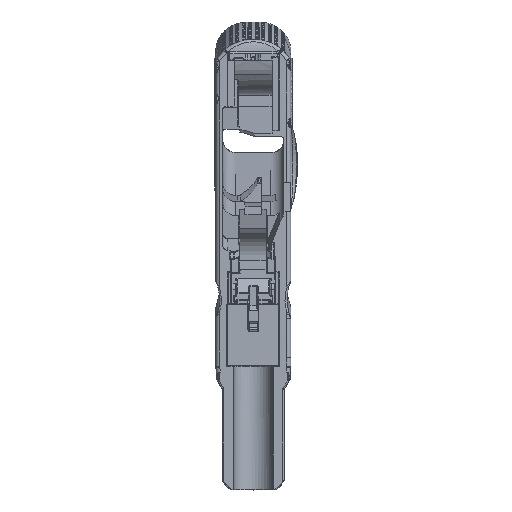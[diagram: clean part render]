
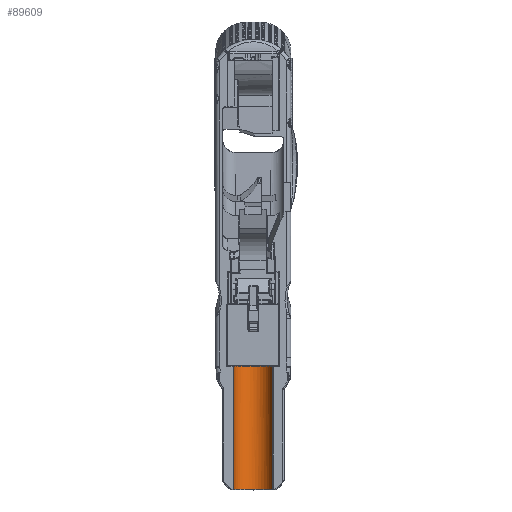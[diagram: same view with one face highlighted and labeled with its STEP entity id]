
A CAD part, top view. The second image highlights one B-rep face of the part: STEP entity #89609.
In plain terms, the highlighted cylindrical face has radius 7.62 mm (diameter 15.24 mm), a partial arc.
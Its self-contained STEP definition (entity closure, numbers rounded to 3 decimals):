
#1249=CYLINDRICAL_SURFACE('',#95398,7.62);
#2247=CIRCLE('',#94868,7.62);
#2250=CIRCLE('',#94872,7.62);
#2254=CIRCLE('',#94876,7.62);
#2475=CIRCLE('',#95399,7.62);
#4872=FACE_OUTER_BOUND('',#10265,.T.);
#10265=EDGE_LOOP('',(#61090,#61091,#61092,#61093,#61094,#61095,#61096,#61097));
#15929=B_SPLINE_CURVE_WITH_KNOTS('',3,(#133860,#133861,#133862,#133863),
 .UNSPECIFIED.,.F.,.F.,(4,4),(0.,0.1),.UNSPECIFIED.);
#15996=B_SPLINE_CURVE_WITH_KNOTS('',3,(#139963,#139964,#139965,#139966),
 .UNSPECIFIED.,.F.,.F.,(4,4),(-0.1,0.),.UNSPECIFIED.);
#18029=LINE('',#138483,#27326);
#18118=LINE('',#139979,#27415);
#27326=VECTOR('',#104218,10.);
#27415=VECTOR('',#104623,10.);
#36746=VERTEX_POINT('',#132628);
#36834=VERTEX_POINT('',#133801);
#36835=VERTEX_POINT('',#133803);
#36836=VERTEX_POINT('',#133808);
#36837=VERTEX_POINT('',#133831);
#37235=VERTEX_POINT('',#138482);
#37351=VERTEX_POINT('',#139960);
#37355=VERTEX_POINT('',#139978);
#45784=EDGE_CURVE('',#36834,#36835,#2247,.T.);
#45787=EDGE_CURVE('',#36835,#36836,#2250,.T.);
#45791=EDGE_CURVE('',#36836,#36837,#2254,.T.);
#45793=EDGE_CURVE('',#36837,#36746,#15929,.T.);
#46393=EDGE_CURVE('',#36746,#37235,#18029,.T.);
#46598=EDGE_CURVE('',#37351,#36834,#15996,.T.);
#46603=EDGE_CURVE('',#37355,#37351,#18118,.T.);
#46604=EDGE_CURVE('',#37235,#37355,#2475,.T.);
#61090=ORIENTED_EDGE('',*,*,#46603,.F.);
#61091=ORIENTED_EDGE('',*,*,#46604,.F.);
#61092=ORIENTED_EDGE('',*,*,#46393,.F.);
#61093=ORIENTED_EDGE('',*,*,#45793,.F.);
#61094=ORIENTED_EDGE('',*,*,#45791,.F.);
#61095=ORIENTED_EDGE('',*,*,#45787,.F.);
#61096=ORIENTED_EDGE('',*,*,#45784,.F.);
#61097=ORIENTED_EDGE('',*,*,#46598,.F.);
#89609=ADVANCED_FACE('',(#4872),#1249,.F.);
#94868=AXIS2_PLACEMENT_3D('',#133804,#103093,#103094);
#94872=AXIS2_PLACEMENT_3D('',#133809,#103101,#103102);
#94876=AXIS2_PLACEMENT_3D('',#133835,#103109,#103110);
#95398=AXIS2_PLACEMENT_3D('',#139977,#104621,#104622);
#95399=AXIS2_PLACEMENT_3D('',#139980,#104624,#104625);
#103093=DIRECTION('center_axis',(0.04,0.999,-0.013));
#103094=DIRECTION('ref_axis',(0.949,-0.042,-0.313));
#103101=DIRECTION('center_axis',(0.,1.,0.));
#103102=DIRECTION('ref_axis',(0.,0.,
-1.));
#103109=DIRECTION('center_axis',(-0.04,0.999,
-0.013));
#103110=DIRECTION('ref_axis',(-0.991,-0.041,-0.127));
#104218=DIRECTION('',(0.,1.,0.));
#104621=DIRECTION('center_axis',(0.,1.,0.));
#104622=DIRECTION('ref_axis',(1.,0.,0.));
#104623=DIRECTION('',(0.,-1.,0.));
#104624=DIRECTION('center_axis',(0.,-1.,0.));
#104625=DIRECTION('ref_axis',(0.,0.,
-1.));
#132628=CARTESIAN_POINT('',(-7.62,-74.215,70.65));
#133801=CARTESIAN_POINT('',(7.558,-74.219,69.684));
#133803=CARTESIAN_POINT('',(7.236,-74.225,68.261));
#133804=CARTESIAN_POINT('Origin',(0.007,-73.908,
70.647));
#133808=CARTESIAN_POINT('',(-7.236,-74.225,68.262));
#133809=CARTESIAN_POINT('Origin',(0.,-74.225,
70.65));
#133831=CARTESIAN_POINT('',(-7.558,-74.219,69.684));
#133835=CARTESIAN_POINT('Origin',(-0.006,-73.908,
70.647));
#133860=CARTESIAN_POINT('Ctrl Pts',(-7.558,-74.219,
69.684));
#133861=CARTESIAN_POINT('Ctrl Pts',(-7.599,-74.217,
70.004));
#133862=CARTESIAN_POINT('Ctrl Pts',(-7.62,-74.215,
70.327));
#133863=CARTESIAN_POINT('Ctrl Pts',(-7.62,-74.215,
70.65));
#138482=CARTESIAN_POINT('',(-7.62,-26.317,70.65));
#138483=CARTESIAN_POINT('',(-7.62,-74.479,70.65));
#139960=CARTESIAN_POINT('',(7.62,-74.215,70.65));
#139963=CARTESIAN_POINT('Ctrl Pts',(7.62,-74.215,70.65));
#139964=CARTESIAN_POINT('Ctrl Pts',(7.62,-74.215,70.327));
#139965=CARTESIAN_POINT('Ctrl Pts',(7.599,-74.217,70.004));
#139966=CARTESIAN_POINT('Ctrl Pts',(7.558,-74.219,69.684));
#139977=CARTESIAN_POINT('Origin',(0.,-74.479,
70.65));
#139978=CARTESIAN_POINT('',(7.62,-26.317,70.65));
#139979=CARTESIAN_POINT('',(7.62,-31.909,70.65));
#139980=CARTESIAN_POINT('Origin',(0.,-26.317,
70.65));
